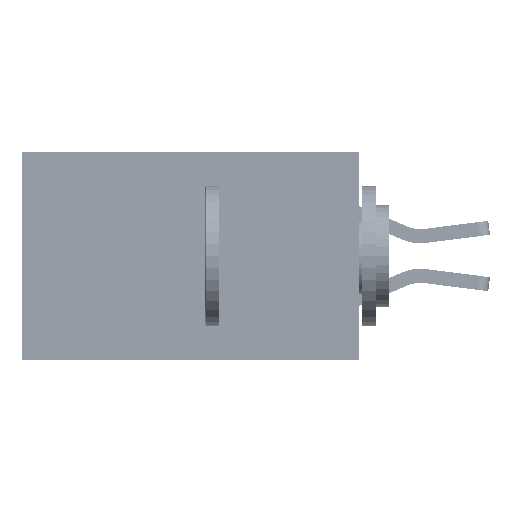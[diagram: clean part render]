
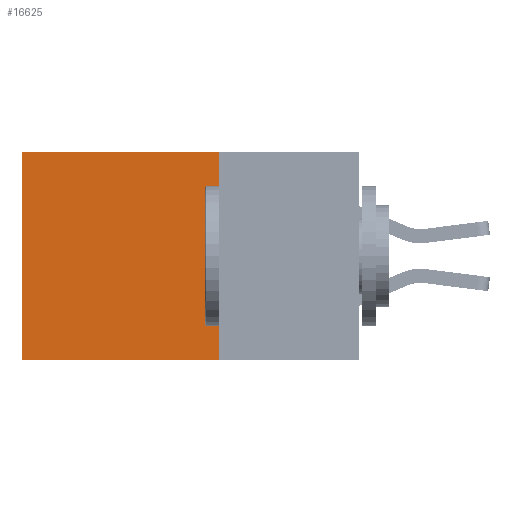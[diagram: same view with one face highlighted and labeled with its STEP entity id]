
A CAD part, left-side view. The second image highlights one B-rep face of the part: STEP entity #16625.
In plain terms, the highlighted planar face has unit normal (-1, 0, 0).
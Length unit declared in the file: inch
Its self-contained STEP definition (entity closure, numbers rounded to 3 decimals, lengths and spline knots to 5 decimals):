
#218 = ORIENTED_EDGE ( 'NONE', *, *, #8436, .F. ) ;
#722 = CARTESIAN_POINT ( 'NONE',  ( 0.2875, 0.6, 0. ) ) ;
#908 = VECTOR ( 'NONE', #45513, 39.37008 ) ;
#1104 = PLANE ( 'NONE',  #32304 ) ;
#1390 = EDGE_CURVE ( 'NONE', #43955, #12553, #39104, .T. ) ;
#3484 = EDGE_CURVE ( 'NONE', #12553, #44466, #45234, .T. ) ;
#3534 = CARTESIAN_POINT ( 'NONE',  ( 0.2875, 0.25, 0. ) ) ;
#7158 = LINE ( 'NONE', #31699, #908 ) ;
#7913 = DIRECTION ( 'NONE',  ( 0., 0., -1. ) ) ;
#8436 = EDGE_CURVE ( 'NONE', #31599, #44466, #7158, .T. ) ;
#9316 = LINE ( 'NONE', #46895, #37049 ) ;
#9970 = DIRECTION ( 'NONE',  ( 0., 0., -1. ) ) ;
#10549 = ORIENTED_EDGE ( 'NONE', *, *, #34412, .F. ) ;
#11107 = FACE_OUTER_BOUND ( 'NONE', #15915, .T. ) ;
#12184 = ORIENTED_EDGE ( 'NONE', *, *, #1390, .T. ) ;
#12553 = VERTEX_POINT ( 'NONE', #722 ) ;
#15915 = EDGE_LOOP ( 'NONE', ( #32185, #218, #10549, #12184 ) ) ;
#16625 = ADVANCED_FACE ( 'NONE', ( #11107 ), #1104, .F. ) ;
#22797 = CARTESIAN_POINT ( 'NONE',  ( 0.2875, 0.25, -0.37 ) ) ;
#23528 = CARTESIAN_POINT ( 'NONE',  ( 0.2875, 0.6, -0.37 ) ) ;
#26337 = CARTESIAN_POINT ( 'NONE',  ( 0.2875, 0.25, 0. ) ) ;
#31599 = VERTEX_POINT ( 'NONE', #22797 ) ;
#31699 = CARTESIAN_POINT ( 'NONE',  ( 0.2875, 0.25, -0.37 ) ) ;
#32185 = ORIENTED_EDGE ( 'NONE', *, *, #3484, .T. ) ;
#32304 = AXIS2_PLACEMENT_3D ( 'NONE', #44490, #44179, #7913 ) ;
#34412 = EDGE_CURVE ( 'NONE', #43955, #31599, #9316, .T. ) ;
#34588 = VECTOR ( 'NONE', #37860, 39.37008 ) ;
#35586 = VECTOR ( 'NONE', #9970, 39.37008 ) ;
#37049 = VECTOR ( 'NONE', #43211, 39.37008 ) ;
#37860 = DIRECTION ( 'NONE',  ( 0., 1., 0. ) ) ;
#39104 = LINE ( 'NONE', #26337, #34588 ) ;
#39231 = CARTESIAN_POINT ( 'NONE',  ( 0.2875, 0.6, 0. ) ) ;
#43211 = DIRECTION ( 'NONE',  ( 0., 0., -1. ) ) ;
#43955 = VERTEX_POINT ( 'NONE', #3534 ) ;
#44179 = DIRECTION ( 'NONE',  ( 1., 0., 0. ) ) ;
#44466 = VERTEX_POINT ( 'NONE', #23528 ) ;
#44490 = CARTESIAN_POINT ( 'NONE',  ( 0.2875, 0.25, 0. ) ) ;
#45234 = LINE ( 'NONE', #39231, #35586 ) ;
#45513 = DIRECTION ( 'NONE',  ( 0., 1., 0. ) ) ;
#46895 = CARTESIAN_POINT ( 'NONE',  ( 0.2875, 0.25, 0. ) ) ;
